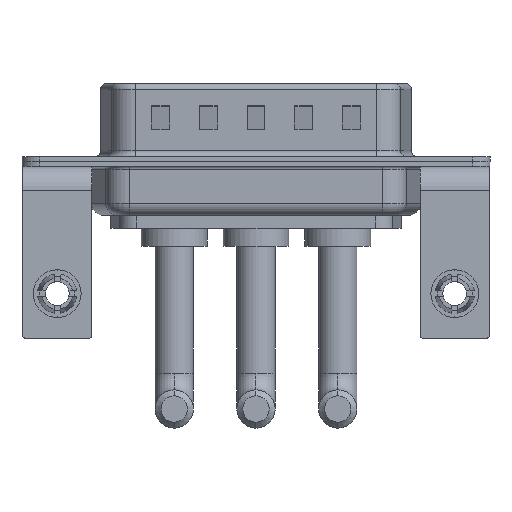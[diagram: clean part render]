
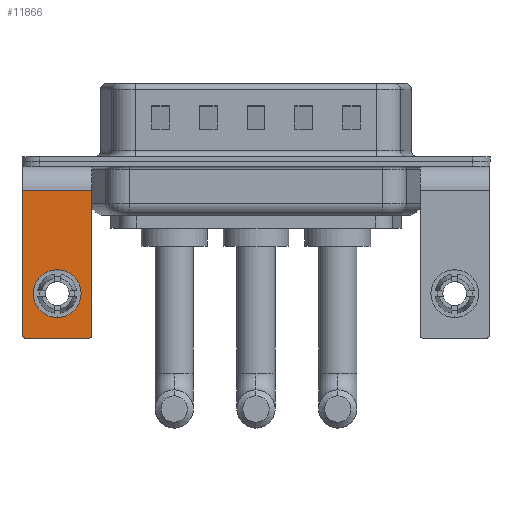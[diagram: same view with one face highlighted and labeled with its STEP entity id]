
A CAD part, front view. The second image highlights one B-rep face of the part: STEP entity #11866.
In plain terms, the highlighted planar face has unit normal (0, -1, 0).
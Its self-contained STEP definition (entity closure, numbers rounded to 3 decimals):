
#67 = CARTESIAN_POINT ( 'NONE',  ( 2.65, -6.25, -14.8 ) ) ;
#615 = VERTEX_POINT ( 'NONE', #10884 ) ;
#652 = VERTEX_POINT ( 'NONE', #1571 ) ;
#1113 = CARTESIAN_POINT ( 'NONE',  ( 2.65, -6.25, -14.55 ) ) ;
#1181 = ORIENTED_EDGE ( 'NONE', *, *, #4944, .F. ) ;
#1571 = CARTESIAN_POINT ( 'NONE',  ( 2.9, -6.25, -14.55 ) ) ;
#2034 = CARTESIAN_POINT ( 'NONE',  ( 0., -6.25, -11.07 ) ) ;
#2057 = EDGE_CURVE ( 'NONE', #5871, #652, #13755, .T. ) ;
#2377 = CIRCLE ( 'NONE', #3834, 2. ) ;
#3134 = EDGE_CURVE ( 'NONE', #16485, #652, #16740, .T. ) ;
#3243 = DIRECTION ( 'NONE',  ( 0., 0., 1. ) ) ;
#3354 = CARTESIAN_POINT ( 'NONE',  ( 2.9, -6.25, -2.4 ) ) ;
#3556 = VERTEX_POINT ( 'NONE', #5423 ) ;
#3834 = AXIS2_PLACEMENT_3D ( 'NONE', #13603, #3997, #10744 ) ;
#3919 = DIRECTION ( 'NONE',  ( 0., 0., -1. ) ) ;
#3997 = DIRECTION ( 'NONE',  ( 0., 1., 0. ) ) ;
#4526 = DIRECTION ( 'NONE',  ( 0., -1., 0. ) ) ;
#4640 = LINE ( 'NONE', #3354, #6740 ) ;
#4732 = EDGE_CURVE ( 'NONE', #5871, #615, #4640, .T. ) ;
#4944 = EDGE_CURVE ( 'NONE', #16485, #15258, #9711, .T. ) ;
#5423 = CARTESIAN_POINT ( 'NONE',  ( -2.9, -6.25, -14.55 ) ) ;
#5799 = EDGE_CURVE ( 'NONE', #14772, #9851, #2377, .T. ) ;
#5813 = EDGE_LOOP ( 'NONE', ( #18112, #15079 ) ) ;
#5871 = VERTEX_POINT ( 'NONE', #8065 ) ;
#6687 = LINE ( 'NONE', #15182, #12889 ) ;
#6740 = VECTOR ( 'NONE', #17486, 1000. ) ;
#6912 = DIRECTION ( 'NONE',  ( 0., 0., 1. ) ) ;
#7069 = CIRCLE ( 'NONE', #15918, 2. ) ;
#7128 = CARTESIAN_POINT ( 'NONE',  ( 2.9, -6.25, -14.8 ) ) ;
#7303 = FACE_OUTER_BOUND ( 'NONE', #16160, .T. ) ;
#7485 = DIRECTION ( 'NONE',  ( 0., 1., 0. ) ) ;
#8065 = CARTESIAN_POINT ( 'NONE',  ( 2.9, -6.25, -2.4 ) ) ;
#8090 = ORIENTED_EDGE ( 'NONE', *, *, #2057, .F. ) ;
#8532 = ORIENTED_EDGE ( 'NONE', *, *, #3134, .T. ) ;
#8613 = ORIENTED_EDGE ( 'NONE', *, *, #4732, .T. ) ;
#8679 = CARTESIAN_POINT ( 'NONE',  ( -2.65, -6.25, -14.55 ) ) ;
#9174 = ORIENTED_EDGE ( 'NONE', *, *, #17952, .T. ) ;
#9711 = LINE ( 'NONE', #7128, #17667 ) ;
#9851 = VERTEX_POINT ( 'NONE', #15106 ) ;
#10744 = DIRECTION ( 'NONE',  ( 0., 0., 1. ) ) ;
#10884 = CARTESIAN_POINT ( 'NONE',  ( -2.9, -6.25, -2.4 ) ) ;
#10980 = DIRECTION ( 'NONE',  ( 0., -1., 0. ) ) ;
#11212 = AXIS2_PLACEMENT_3D ( 'NONE', #8679, #4526, #15887 ) ;
#11472 = PLANE ( 'NONE',  #11604 ) ;
#11604 = AXIS2_PLACEMENT_3D ( 'NONE', #17466, #7485, #3243 ) ;
#11866 = ADVANCED_FACE ( 'NONE', ( #14409, #7303 ), #11472, .F. ) ;
#12763 = DIRECTION ( 'NONE',  ( -1., 0., 0. ) ) ;
#12850 = ORIENTED_EDGE ( 'NONE', *, *, #14860, .T. ) ;
#12889 = VECTOR ( 'NONE', #3919, 1000. ) ;
#12970 = CIRCLE ( 'NONE', #11212, 0.25 ) ;
#13141 = CARTESIAN_POINT ( 'NONE',  ( -2.65, -6.25, -14.8 ) ) ;
#13284 = DIRECTION ( 'NONE',  ( 0., 1., 0. ) ) ;
#13603 = CARTESIAN_POINT ( 'NONE',  ( 0., -6.25, -11.07 ) ) ;
#13755 = LINE ( 'NONE', #18022, #15557 ) ;
#14075 = AXIS2_PLACEMENT_3D ( 'NONE', #1113, #10980, #6912 ) ;
#14409 = FACE_BOUND ( 'NONE', #5813, .T. ) ;
#14772 = VERTEX_POINT ( 'NONE', #14904 ) ;
#14860 = EDGE_CURVE ( 'NONE', #615, #3556, #6687, .T. ) ;
#14904 = CARTESIAN_POINT ( 'NONE',  ( 0., -6.25, -13.07 ) ) ;
#15079 = ORIENTED_EDGE ( 'NONE', *, *, #17534, .T. ) ;
#15106 = CARTESIAN_POINT ( 'NONE',  ( 0., -6.25, -9.07 ) ) ;
#15182 = CARTESIAN_POINT ( 'NONE',  ( -2.9, -6.25, -2.4 ) ) ;
#15258 = VERTEX_POINT ( 'NONE', #13141 ) ;
#15557 = VECTOR ( 'NONE', #16640, 1000. ) ;
#15887 = DIRECTION ( 'NONE',  ( 0., 0., 1. ) ) ;
#15918 = AXIS2_PLACEMENT_3D ( 'NONE', #2034, #13284, #17530 ) ;
#16160 = EDGE_LOOP ( 'NONE', ( #12850, #9174, #1181, #8532, #8090, #8613 ) ) ;
#16485 = VERTEX_POINT ( 'NONE', #67 ) ;
#16640 = DIRECTION ( 'NONE',  ( 0., 0., -1. ) ) ;
#16740 = CIRCLE ( 'NONE', #14075, 0.25 ) ;
#17466 = CARTESIAN_POINT ( 'NONE',  ( 2.9, -6.25, -2.4 ) ) ;
#17486 = DIRECTION ( 'NONE',  ( -1., 0., 0. ) ) ;
#17530 = DIRECTION ( 'NONE',  ( 0., 0., 1. ) ) ;
#17534 = EDGE_CURVE ( 'NONE', #9851, #14772, #7069, .T. ) ;
#17667 = VECTOR ( 'NONE', #12763, 1000. ) ;
#17952 = EDGE_CURVE ( 'NONE', #3556, #15258, #12970, .T. ) ;
#18022 = CARTESIAN_POINT ( 'NONE',  ( 2.9, -6.25, -2.4 ) ) ;
#18112 = ORIENTED_EDGE ( 'NONE', *, *, #5799, .T. ) ;
